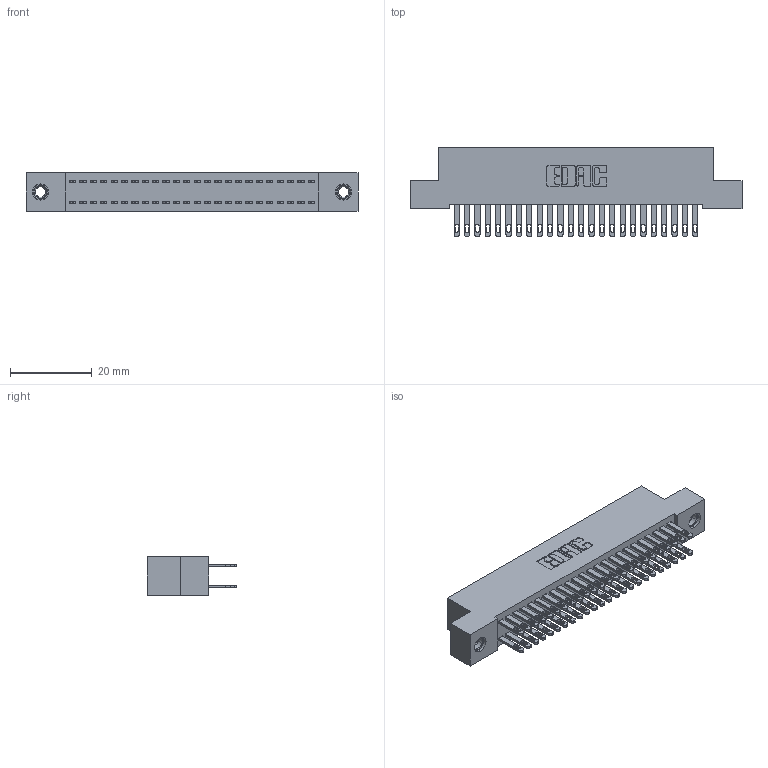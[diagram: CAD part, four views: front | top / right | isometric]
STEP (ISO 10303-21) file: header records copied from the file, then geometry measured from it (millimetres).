
FILE_DESCRIPTION (( 'STEP AP203' ), '1' );
FILE_NAME ('892-048-500-207.STEP', '2020-09-21T17:36:03', ( '' ), ( '' ), 'SwSTEP 2.0', 'SolidWorks 2020', '' );
FILE_SCHEMA (( 'CONFIG_CONTROL_DESIGN' ));
Length unit declared in the file: inch
Products named in the file (4): 892-048-500-207; 345-292-001_345-293-100; 842 Part_TI; 345-250-001_345-250-005-103
Assembly tree (51 placements, depth 2):
  892-048-500-207
    842 Part_TI
    345-292-001_345-293-100  x48
    345-250-001_345-250-005-103  x2
Bounding box: 81.28 x 21.85 x 9.4 mm (x, y, z)
Volume: 7351.8 mm3; surface area: 12008.7 mm2
Topology: 51 solids, 51 shells, 2474 faces, 7491 edges, 4986 vertices
Faces by surface type: plane 1538, cylinder 920, cone 12, torus 4
Entity records: 18752 total; most frequent: CARTESIAN_POINT 3109, ORIENTED_EDGE 3038, DIRECTION 2721, EDGE_CURVE 1519, VECTOR 1367, LINE 1367, VERTEX_POINT 1008, AXIS2_PLACEMENT_3D 677
